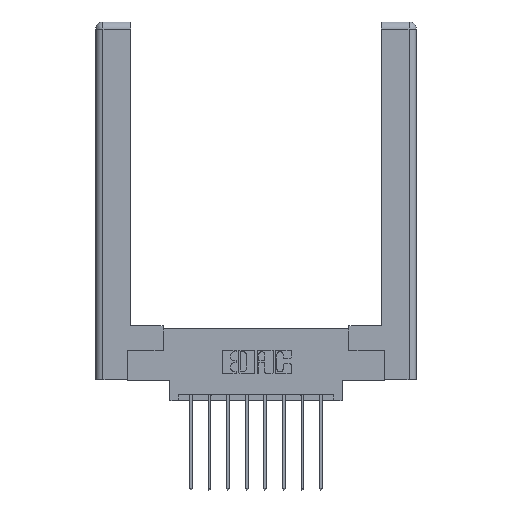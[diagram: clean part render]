
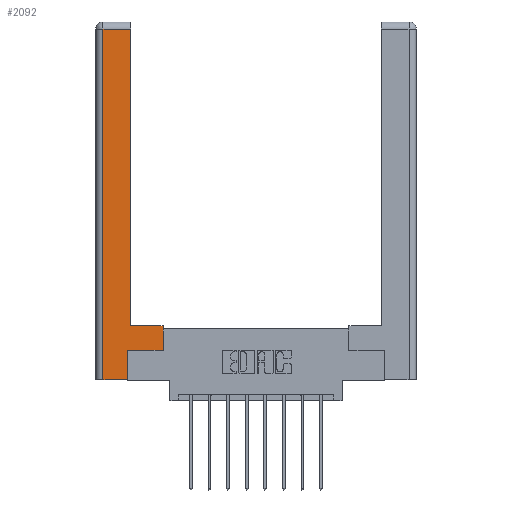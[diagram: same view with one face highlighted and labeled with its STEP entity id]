
A CAD part, top view. The second image highlights one B-rep face of the part: STEP entity #2092.
In plain terms, the highlighted planar face has unit normal (0, 0, 1).
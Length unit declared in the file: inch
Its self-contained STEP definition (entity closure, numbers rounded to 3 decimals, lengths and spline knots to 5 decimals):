
#47 = VERTEX_POINT ( 'NONE', #2789 ) ;
#208 = VECTOR ( 'NONE', #670, 39.37008 ) ;
#409 = DIRECTION ( 'NONE',  ( 1., 0., 0. ) ) ;
#670 = DIRECTION ( 'NONE',  ( 0., -1., 0. ) ) ;
#1187 = LINE ( 'NONE', #3993, #7350 ) ;
#1256 = ORIENTED_EDGE ( 'NONE', *, *, #5224, .T. ) ;
#1289 = DIRECTION ( 'NONE',  ( 0., 1., 0. ) ) ;
#1315 = ORIENTED_EDGE ( 'NONE', *, *, #6360, .T. ) ;
#1766 = CARTESIAN_POINT ( 'NONE',  ( 0.0615, 2.94, 0. ) ) ;
#2062 = VECTOR ( 'NONE', #4779, 39.37008 ) ;
#2092 = ADVANCED_FACE ( 'NONE', ( #7042 ), #6472, .F. ) ;
#2155 = ORIENTED_EDGE ( 'NONE', *, *, #9380, .T. ) ;
#2374 = EDGE_CURVE ( 'NONE', #5988, #8604, #10629, .T. ) ;
#2789 = CARTESIAN_POINT ( 'NONE',  ( 0.265, 0.245, 0. ) ) ;
#2993 = CARTESIAN_POINT ( 'NONE',  ( 0.295, 2.94, 0. ) ) ;
#3146 = DIRECTION ( 'NONE',  ( 0., 1., 0. ) ) ;
#3328 = CARTESIAN_POINT ( 'NONE',  ( 0.295, 0.45, 0. ) ) ;
#3918 = LINE ( 'NONE', #7216, #6825 ) ;
#3946 = DIRECTION ( 'NONE',  ( 1., 0., 0. ) ) ;
#3993 = CARTESIAN_POINT ( 'NONE',  ( 0.565, 0.245, 0. ) ) ;
#4163 = CARTESIAN_POINT ( 'NONE',  ( 0.565, 0.245, 0. ) ) ;
#4517 = DIRECTION ( 'NONE',  ( 0., 1., 0. ) ) ;
#4779 = DIRECTION ( 'NONE',  ( -1., 0., 0. ) ) ;
#4900 = VECTOR ( 'NONE', #5055, 39.37008 ) ;
#5055 = DIRECTION ( 'NONE',  ( -1., 0., 0. ) ) ;
#5067 = LINE ( 'NONE', #8418, #12991 ) ;
#5103 = ORIENTED_EDGE ( 'NONE', *, *, #2374, .T. ) ;
#5224 = EDGE_CURVE ( 'NONE', #9250, #5988, #5792, .T. ) ;
#5381 = CARTESIAN_POINT ( 'NONE',  ( 0., 0., 0. ) ) ;
#5412 = CARTESIAN_POINT ( 'NONE',  ( 0.0615, 2.94, 0. ) ) ;
#5558 = LINE ( 'NONE', #8074, #4900 ) ;
#5792 = LINE ( 'NONE', #1766, #2062 ) ;
#5988 = VERTEX_POINT ( 'NONE', #5412 ) ;
#6059 = EDGE_CURVE ( 'NONE', #11287, #9250, #10516, .T. ) ;
#6292 = ORIENTED_EDGE ( 'NONE', *, *, #10672, .T. ) ;
#6317 = DIRECTION ( 'NONE',  ( -1., 0., 0. ) ) ;
#6360 = EDGE_CURVE ( 'NONE', #8604, #10842, #9184, .T. ) ;
#6472 = PLANE ( 'NONE',  #9065 ) ;
#6825 = VECTOR ( 'NONE', #3146, 39.37008 ) ;
#6908 = VECTOR ( 'NONE', #409, 39.37008 ) ;
#7042 = FACE_OUTER_BOUND ( 'NONE', #9511, .T. ) ;
#7216 = CARTESIAN_POINT ( 'NONE',  ( 0.565, 0.45, 0. ) ) ;
#7350 = VECTOR ( 'NONE', #3946, 39.37008 ) ;
#8074 = CARTESIAN_POINT ( 'NONE',  ( 0.295, 0.45, 0. ) ) ;
#8418 = CARTESIAN_POINT ( 'NONE',  ( 0.265, 0.245, 0. ) ) ;
#8553 = CARTESIAN_POINT ( 'NONE',  ( 0.0615, 0., 0. ) ) ;
#8555 = CARTESIAN_POINT ( 'NONE',  ( 0.295, 3., 0. ) ) ;
#8570 = ORIENTED_EDGE ( 'NONE', *, *, #11488, .T. ) ;
#8604 = VERTEX_POINT ( 'NONE', #8553 ) ;
#8880 = CARTESIAN_POINT ( 'NONE',  ( 0.565, 0.45, 0. ) ) ;
#9065 = AXIS2_PLACEMENT_3D ( 'NONE', #5381, #12694, #6317 ) ;
#9106 = CARTESIAN_POINT ( 'NONE',  ( 0.265, 0., 0. ) ) ;
#9113 = VERTEX_POINT ( 'NONE', #8880 ) ;
#9184 = LINE ( 'NONE', #11526, #6908 ) ;
#9250 = VERTEX_POINT ( 'NONE', #2993 ) ;
#9380 = EDGE_CURVE ( 'NONE', #10842, #47, #5067, .T. ) ;
#9511 = EDGE_LOOP ( 'NONE', ( #11821, #1256, #5103, #1315, #2155, #10206, #6292, #8570 ) ) ;
#9525 = VECTOR ( 'NONE', #1289, 39.37008 ) ;
#9639 = CARTESIAN_POINT ( 'NONE',  ( 0.0615, 0., 0. ) ) ;
#10206 = ORIENTED_EDGE ( 'NONE', *, *, #11421, .T. ) ;
#10516 = LINE ( 'NONE', #8555, #9525 ) ;
#10629 = LINE ( 'NONE', #9639, #208 ) ;
#10672 = EDGE_CURVE ( 'NONE', #11632, #9113, #3918, .T. ) ;
#10842 = VERTEX_POINT ( 'NONE', #9106 ) ;
#11287 = VERTEX_POINT ( 'NONE', #3328 ) ;
#11421 = EDGE_CURVE ( 'NONE', #47, #11632, #1187, .T. ) ;
#11488 = EDGE_CURVE ( 'NONE', #9113, #11287, #5558, .T. ) ;
#11526 = CARTESIAN_POINT ( 'NONE',  ( 0.265, 0., 0. ) ) ;
#11632 = VERTEX_POINT ( 'NONE', #4163 ) ;
#11821 = ORIENTED_EDGE ( 'NONE', *, *, #6059, .T. ) ;
#12694 = DIRECTION ( 'NONE',  ( 0., 0., -1. ) ) ;
#12991 = VECTOR ( 'NONE', #4517, 39.37008 ) ;
